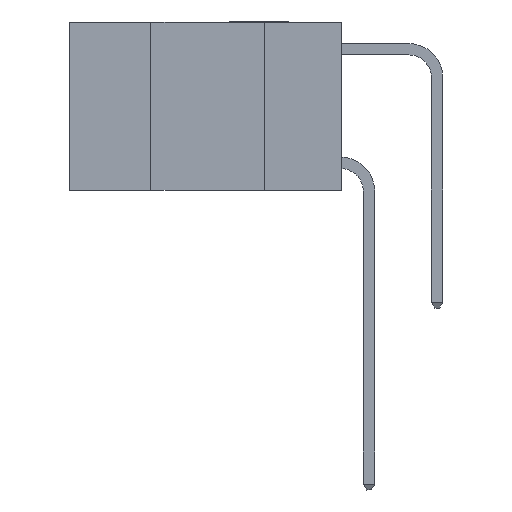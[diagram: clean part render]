
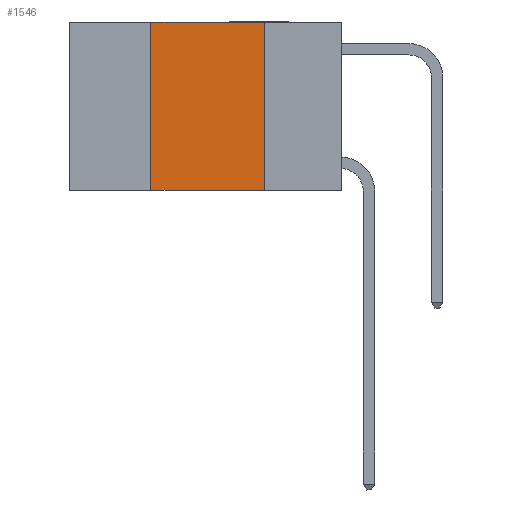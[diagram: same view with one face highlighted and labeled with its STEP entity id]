
A CAD part, left-side view. The second image highlights one B-rep face of the part: STEP entity #1546.
In plain terms, the highlighted planar face has unit normal (-1, 0, 0).
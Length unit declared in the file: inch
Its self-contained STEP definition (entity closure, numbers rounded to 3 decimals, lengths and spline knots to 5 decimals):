
#896 = EDGE_CURVE ( 'NONE', #4218, #7077, #1908, .T. ) ;
#1254 = DIRECTION ( 'NONE',  ( 1., 0., 0. ) ) ;
#1546 = ADVANCED_FACE ( 'NONE', ( #4978 ), #10547, .F. ) ;
#1908 = LINE ( 'NONE', #2498, #10549 ) ;
#1909 = DIRECTION ( 'NONE',  ( 0., 0., 1. ) ) ;
#1949 = VECTOR ( 'NONE', #8700, 39.37008 ) ;
#2012 = CARTESIAN_POINT ( 'NONE',  ( 0., 0.6, -0.37 ) ) ;
#2246 = LINE ( 'NONE', #6226, #1949 ) ;
#2498 = CARTESIAN_POINT ( 'NONE',  ( 0., 0.17, 0. ) ) ;
#2631 = DIRECTION ( 'NONE',  ( 0., 0., -1. ) ) ;
#2746 = VERTEX_POINT ( 'NONE', #8154 ) ;
#2927 = CARTESIAN_POINT ( 'NONE',  ( 0., 0.42, -0.37 ) ) ;
#4136 = EDGE_LOOP ( 'NONE', ( #5902, #6041, #6143, #6188 ) ) ;
#4218 = VERTEX_POINT ( 'NONE', #4573 ) ;
#4573 = CARTESIAN_POINT ( 'NONE',  ( 0., 0.17, 0. ) ) ;
#4978 = FACE_OUTER_BOUND ( 'NONE', #4136, .T. ) ;
#5902 = ORIENTED_EDGE ( 'NONE', *, *, #896, .F. ) ;
#6041 = ORIENTED_EDGE ( 'NONE', *, *, #6067, .F. ) ;
#6067 = EDGE_CURVE ( 'NONE', #2746, #4218, #2246, .T. ) ;
#6085 = VECTOR ( 'NONE', #1909, 39.37008 ) ;
#6143 = ORIENTED_EDGE ( 'NONE', *, *, #6166, .F. ) ;
#6166 = EDGE_CURVE ( 'NONE', #6266, #2746, #6348, .T. ) ;
#6188 = ORIENTED_EDGE ( 'NONE', *, *, #10872, .T. ) ;
#6226 = CARTESIAN_POINT ( 'NONE',  ( 0., 0.6, 0. ) ) ;
#6266 = VERTEX_POINT ( 'NONE', #2927 ) ;
#6348 = LINE ( 'NONE', #10281, #6085 ) ;
#6529 = LINE ( 'NONE', #2012, #8703 ) ;
#6598 = CARTESIAN_POINT ( 'NONE',  ( 0., 0.6, 0. ) ) ;
#7077 = VERTEX_POINT ( 'NONE', #7880 ) ;
#7454 = DIRECTION ( 'NONE',  ( 0., 0., -1. ) ) ;
#7880 = CARTESIAN_POINT ( 'NONE',  ( 0., 0.17, -0.37 ) ) ;
#8154 = CARTESIAN_POINT ( 'NONE',  ( 0., 0.42, 0. ) ) ;
#8442 = AXIS2_PLACEMENT_3D ( 'NONE', #6598, #1254, #7454 ) ;
#8700 = DIRECTION ( 'NONE',  ( 0., -1., 0. ) ) ;
#8703 = VECTOR ( 'NONE', #10367, 39.37008 ) ;
#10281 = CARTESIAN_POINT ( 'NONE',  ( 0., 0.42, 0. ) ) ;
#10367 = DIRECTION ( 'NONE',  ( 0., -1., 0. ) ) ;
#10547 = PLANE ( 'NONE',  #8442 ) ;
#10549 = VECTOR ( 'NONE', #2631, 39.37008 ) ;
#10872 = EDGE_CURVE ( 'NONE', #6266, #7077, #6529, .T. ) ;
